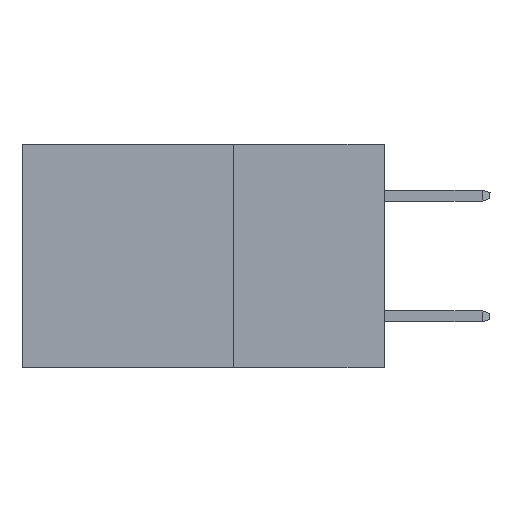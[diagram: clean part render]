
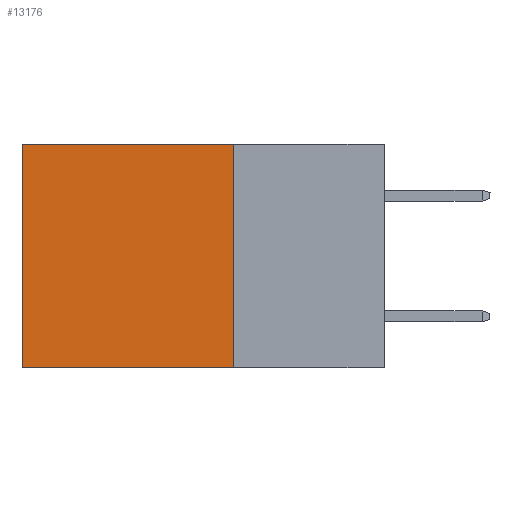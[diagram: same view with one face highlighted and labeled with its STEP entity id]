
A CAD part, left-side view. The second image highlights one B-rep face of the part: STEP entity #13176.
In plain terms, the highlighted planar face has unit normal (-1, 0, 0).
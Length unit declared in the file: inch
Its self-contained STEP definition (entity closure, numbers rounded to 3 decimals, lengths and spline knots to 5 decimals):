
#63 = VERTEX_POINT ( 'NONE', #8349 ) ;
#555 = DIRECTION ( 'NONE',  ( 1., 0., 0. ) ) ;
#870 = VERTEX_POINT ( 'NONE', #2420 ) ;
#1849 = VERTEX_POINT ( 'NONE', #6244 ) ;
#1988 = CARTESIAN_POINT ( 'NONE',  ( 0.298, 0.25, 0. ) ) ;
#2274 = VECTOR ( 'NONE', #9721, 39.37008 ) ;
#2420 = CARTESIAN_POINT ( 'NONE',  ( 0.298, 0.25, 0. ) ) ;
#3170 = VERTEX_POINT ( 'NONE', #3179 ) ;
#3179 = CARTESIAN_POINT ( 'NONE',  ( 0.298, 0.25, -0.37 ) ) ;
#4226 = LINE ( 'NONE', #21720, #4509 ) ;
#4509 = VECTOR ( 'NONE', #10983, 39.37008 ) ;
#5291 = EDGE_CURVE ( 'NONE', #870, #3170, #20351, .T. ) ;
#5863 = CARTESIAN_POINT ( 'NONE',  ( 0.298, 0.25, 0. ) ) ;
#6244 = CARTESIAN_POINT ( 'NONE',  ( 0.298, 0.6, 0. ) ) ;
#6618 = CARTESIAN_POINT ( 'NONE',  ( 0.298, 0.6, 0. ) ) ;
#7236 = ORIENTED_EDGE ( 'NONE', *, *, #5291, .F. ) ;
#7865 = ORIENTED_EDGE ( 'NONE', *, *, #8764, .F. ) ;
#8287 = LINE ( 'NONE', #6618, #16498 ) ;
#8349 = CARTESIAN_POINT ( 'NONE',  ( 0.298, 0.6, -0.37 ) ) ;
#8764 = EDGE_CURVE ( 'NONE', #3170, #63, #4226, .T. ) ;
#8947 = EDGE_CURVE ( 'NONE', #870, #1849, #16720, .T. ) ;
#9205 = DIRECTION ( 'NONE',  ( 0., 0., -1. ) ) ;
#9721 = DIRECTION ( 'NONE',  ( 0., 1., 0. ) ) ;
#10983 = DIRECTION ( 'NONE',  ( 0., 1., 0. ) ) ;
#12488 = ORIENTED_EDGE ( 'NONE', *, *, #23388, .T. ) ;
#13176 = ADVANCED_FACE ( 'NONE', ( #16618 ), #16718, .F. ) ;
#15633 = DIRECTION ( 'NONE',  ( 0., 0., -1. ) ) ;
#16498 = VECTOR ( 'NONE', #15633, 39.37008 ) ;
#16550 = DIRECTION ( 'NONE',  ( 0., 0., -1. ) ) ;
#16618 = FACE_OUTER_BOUND ( 'NONE', #21967, .T. ) ;
#16718 = PLANE ( 'NONE',  #19024 ) ;
#16720 = LINE ( 'NONE', #18766, #2274 ) ;
#18766 = CARTESIAN_POINT ( 'NONE',  ( 0.298, 0.25, 0. ) ) ;
#19024 = AXIS2_PLACEMENT_3D ( 'NONE', #5863, #555, #16550 ) ;
#19187 = VECTOR ( 'NONE', #9205, 39.37008 ) ;
#19194 = ORIENTED_EDGE ( 'NONE', *, *, #8947, .T. ) ;
#20351 = LINE ( 'NONE', #1988, #19187 ) ;
#21720 = CARTESIAN_POINT ( 'NONE',  ( 0.298, 0.25, -0.37 ) ) ;
#21967 = EDGE_LOOP ( 'NONE', ( #12488, #7865, #7236, #19194 ) ) ;
#23388 = EDGE_CURVE ( 'NONE', #1849, #63, #8287, .T. ) ;
